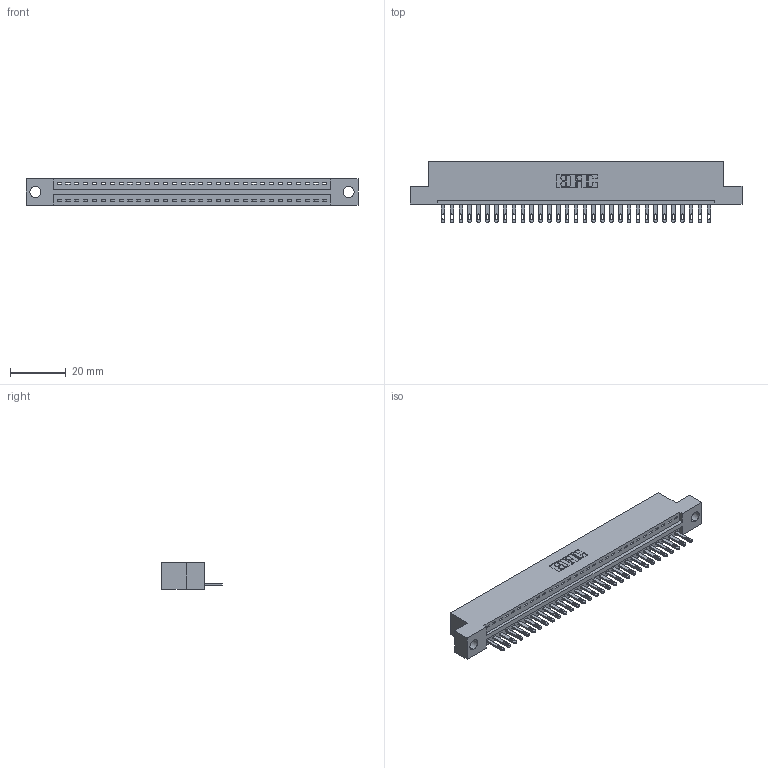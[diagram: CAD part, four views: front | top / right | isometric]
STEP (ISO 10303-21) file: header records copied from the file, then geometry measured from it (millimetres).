
FILE_DESCRIPTION (( 'STEP AP203' ), '1' );
FILE_NAME ('346-031-500-104.STEP', '2022-05-06T16:21:51', ( '' ), ( '' ), 'SwSTEP 2.0', 'SolidWorks 2020', '' );
FILE_SCHEMA (( 'CONFIG_CONTROL_DESIGN' ));
Length unit declared in the file: inch
Products named in the file (3): 346-031-500-104; 346 Part_Flush Mounting Lugs - 0.156 Dia-TH; 345-292-001_345-293-100
Assembly tree (32 placements, depth 2):
  346-031-500-104
    346 Part_Flush Mounting Lugs - 0.156 Dia-TH
    345-292-001_345-293-100  x31
Bounding box: 119 x 21.84 x 9.4 mm (x, y, z)
Volume: 11228.3 mm3; surface area: 13824.7 mm2
Topology: 32 solids, 32 shells, 1810 faces, 5573 edges, 3714 vertices
Faces by surface type: plane 1144, cylinder 666
Entity records: 21069 total; most frequent: CARTESIAN_POINT 3623, ORIENTED_EDGE 3586, DIRECTION 3211, EDGE_CURVE 1793, LINE 1533, VECTOR 1533, VERTEX_POINT 1194, AXIS2_PLACEMENT_3D 839
